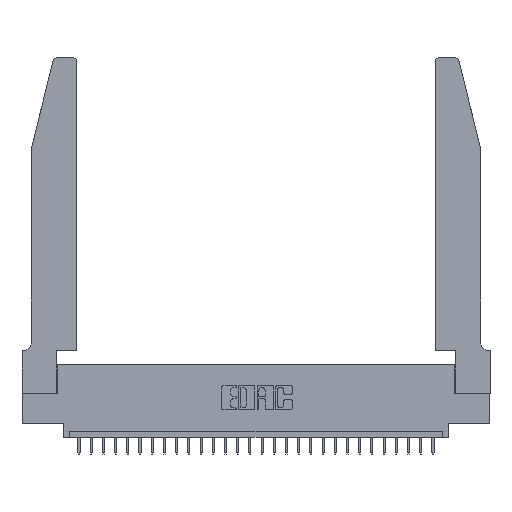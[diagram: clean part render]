
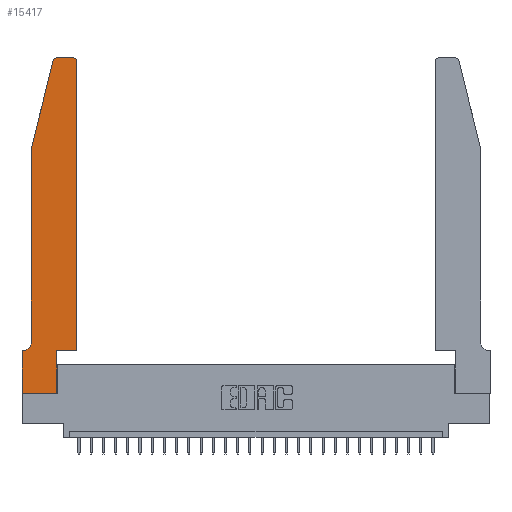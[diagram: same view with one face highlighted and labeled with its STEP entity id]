
A CAD part, top view. The second image highlights one B-rep face of the part: STEP entity #15417.
In plain terms, the highlighted planar face has unit normal (0, 0, 1).
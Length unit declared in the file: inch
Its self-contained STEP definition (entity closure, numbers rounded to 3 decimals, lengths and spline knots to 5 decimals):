
#148 = LINE ( 'NONE', #455, #2557 ) ;
#335 = VERTEX_POINT ( 'NONE', #12648 ) ;
#455 = CARTESIAN_POINT ( 'NONE',  ( 0.2865, 0.35, 0.37 ) ) ;
#881 = CARTESIAN_POINT ( 'NONE',  ( 0.4505, 0.35, 0.37 ) ) ;
#938 = CARTESIAN_POINT ( 'NONE',  ( 0., 0., 0.37 ) ) ;
#1252 = LINE ( 'NONE', #23822, #13345 ) ;
#1320 = LINE ( 'NONE', #881, #8091 ) ;
#1921 = AXIS2_PLACEMENT_3D ( 'NONE', #28984, #17761, #5962 ) ;
#2330 = EDGE_CURVE ( 'NONE', #9192, #14189, #1252, .T. ) ;
#2557 = VECTOR ( 'NONE', #20496, 39.37008 ) ;
#2582 = ORIENTED_EDGE ( 'NONE', *, *, #20068, .T. ) ;
#2652 = EDGE_CURVE ( 'NONE', #6803, #23120, #12443, .T. ) ;
#3059 = CARTESIAN_POINT ( 'NONE',  ( 0.0755, 0.42, 0.37 ) ) ;
#3950 = AXIS2_PLACEMENT_3D ( 'NONE', #7954, #5206, #16710 ) ;
#4109 = DIRECTION ( 'NONE',  ( 1., 0., 0. ) ) ;
#4267 = ORIENTED_EDGE ( 'NONE', *, *, #17699, .T. ) ;
#4570 = VECTOR ( 'NONE', #23733, 39.37008 ) ;
#5076 = EDGE_CURVE ( 'NONE', #20601, #5955, #148, .T. ) ;
#5156 = VERTEX_POINT ( 'NONE', #9600 ) ;
#5206 = DIRECTION ( 'NONE',  ( 0., 0., 1. ) ) ;
#5381 = CARTESIAN_POINT ( 'NONE',  ( 0.0055, 0.35, 0.37 ) ) ;
#5727 = CARTESIAN_POINT ( 'NONE',  ( 0.0755, 0.35, 0.37 ) ) ;
#5955 = VERTEX_POINT ( 'NONE', #24179 ) ;
#5962 = DIRECTION ( 'NONE',  ( 1., 0., 0. ) ) ;
#6500 = CARTESIAN_POINT ( 'NONE',  ( 0.2605, 2.75, 0.37 ) ) ;
#6803 = VERTEX_POINT ( 'NONE', #18201 ) ;
#6940 = DIRECTION ( 'NONE',  ( 1., 0., 0. ) ) ;
#7156 = ORIENTED_EDGE ( 'NONE', *, *, #8086, .T. ) ;
#7325 = VECTOR ( 'NONE', #28973, 39.37008 ) ;
#7926 = VERTEX_POINT ( 'NONE', #19113 ) ;
#7954 = CARTESIAN_POINT ( 'NONE',  ( 0.284, 2.72, 0.37 ) ) ;
#8086 = EDGE_CURVE ( 'NONE', #23120, #17122, #17612, .T. ) ;
#8091 = VECTOR ( 'NONE', #9861, 39.37008 ) ;
#8499 = CARTESIAN_POINT ( 'NONE',  ( 0.2865, 0., 0.37 ) ) ;
#8996 = VERTEX_POINT ( 'NONE', #24468 ) ;
#9074 = ORIENTED_EDGE ( 'NONE', *, *, #9892, .T. ) ;
#9192 = VERTEX_POINT ( 'NONE', #23008 ) ;
#9341 = EDGE_CURVE ( 'NONE', #8996, #9192, #19301, .T. ) ;
#9600 = CARTESIAN_POINT ( 'NONE',  ( 0., 0.35, 0.37 ) ) ;
#9861 = DIRECTION ( 'NONE',  ( 0., 1., 0. ) ) ;
#9892 = EDGE_CURVE ( 'NONE', #10695, #5156, #12097, .T. ) ;
#10539 = AXIS2_PLACEMENT_3D ( 'NONE', #15314, #24321, #4109 ) ;
#10695 = VERTEX_POINT ( 'NONE', #5381 ) ;
#11530 = DIRECTION ( 'NONE',  ( 0., 0., -1. ) ) ;
#12097 = LINE ( 'NONE', #5727, #20634 ) ;
#12145 = LINE ( 'NONE', #938, #12771 ) ;
#12156 = EDGE_CURVE ( 'NONE', #5955, #7926, #13893, .T. ) ;
#12443 = CIRCLE ( 'NONE', #10539, 0.03 ) ;
#12604 = ORIENTED_EDGE ( 'NONE', *, *, #18922, .T. ) ;
#12648 = CARTESIAN_POINT ( 'NONE',  ( 0., 0., 0.37 ) ) ;
#12771 = VECTOR ( 'NONE', #21150, 39.37008 ) ;
#13345 = VECTOR ( 'NONE', #21473, 39.37008 ) ;
#13556 = CARTESIAN_POINT ( 'NONE',  ( 0.4205, 2.75, 0.37 ) ) ;
#13893 = LINE ( 'NONE', #15837, #29138 ) ;
#13999 = ORIENTED_EDGE ( 'NONE', *, *, #9341, .T. ) ;
#14189 = VERTEX_POINT ( 'NONE', #3059 ) ;
#14715 = CARTESIAN_POINT ( 'NONE',  ( 0.0755, 2., 0.37 ) ) ;
#14738 = DIRECTION ( 'NONE',  ( -1., 0., 0. ) ) ;
#15314 = CARTESIAN_POINT ( 'NONE',  ( 0.4205, 2.72, 0.37 ) ) ;
#15417 = ADVANCED_FACE ( 'NONE', ( #24119 ), #26168, .T. ) ;
#15461 = ORIENTED_EDGE ( 'NONE', *, *, #5076, .T. ) ;
#15591 = VECTOR ( 'NONE', #20256, 39.37008 ) ;
#15837 = CARTESIAN_POINT ( 'NONE',  ( 0.4505, 0.35, 0.37 ) ) ;
#15863 = EDGE_LOOP ( 'NONE', ( #7156, #2582, #13999, #16639, #12604, #9074, #22399, #20000, #15461, #22987, #4267, #27259 ) ) ;
#16639 = ORIENTED_EDGE ( 'NONE', *, *, #2330, .T. ) ;
#16710 = DIRECTION ( 'NONE',  ( 1., 0., 0. ) ) ;
#17087 = AXIS2_PLACEMENT_3D ( 'NONE', #17741, #11530, #18045 ) ;
#17122 = VERTEX_POINT ( 'NONE', #22653 ) ;
#17586 = CIRCLE ( 'NONE', #3950, 0.03 ) ;
#17612 = LINE ( 'NONE', #6500, #7325 ) ;
#17699 = EDGE_CURVE ( 'NONE', #7926, #6803, #1320, .T. ) ;
#17741 = CARTESIAN_POINT ( 'NONE',  ( 0.0055, 0.42, 0.37 ) ) ;
#17761 = DIRECTION ( 'NONE',  ( 0., 0., 1. ) ) ;
#18045 = DIRECTION ( 'NONE',  ( -1., 0., 0. ) ) ;
#18201 = CARTESIAN_POINT ( 'NONE',  ( 0.4505, 2.72, 0.37 ) ) ;
#18922 = EDGE_CURVE ( 'NONE', #14189, #10695, #20853, .T. ) ;
#19113 = CARTESIAN_POINT ( 'NONE',  ( 0.4505, 0.35, 0.37 ) ) ;
#19301 = LINE ( 'NONE', #14715, #4570 ) ;
#20000 = ORIENTED_EDGE ( 'NONE', *, *, #24451, .T. ) ;
#20068 = EDGE_CURVE ( 'NONE', #17122, #8996, #17586, .T. ) ;
#20256 = DIRECTION ( 'NONE',  ( 0., -1., 0. ) ) ;
#20496 = DIRECTION ( 'NONE',  ( 0., 1., 0. ) ) ;
#20601 = VERTEX_POINT ( 'NONE', #8499 ) ;
#20634 = VECTOR ( 'NONE', #14738, 39.37008 ) ;
#20853 = CIRCLE ( 'NONE', #17087, 0.07 ) ;
#21150 = DIRECTION ( 'NONE',  ( 1., 0., 0. ) ) ;
#21473 = DIRECTION ( 'NONE',  ( 0., -1., 0. ) ) ;
#22399 = ORIENTED_EDGE ( 'NONE', *, *, #24361, .T. ) ;
#22653 = CARTESIAN_POINT ( 'NONE',  ( 0.284, 2.75, 0.37 ) ) ;
#22987 = ORIENTED_EDGE ( 'NONE', *, *, #12156, .T. ) ;
#23008 = CARTESIAN_POINT ( 'NONE',  ( 0.0755, 2., 0.37 ) ) ;
#23120 = VERTEX_POINT ( 'NONE', #13556 ) ;
#23733 = DIRECTION ( 'NONE',  ( -0.239, -0.971, 0. ) ) ;
#23822 = CARTESIAN_POINT ( 'NONE',  ( 0.0755, 2., 0.37 ) ) ;
#24119 = FACE_OUTER_BOUND ( 'NONE', #15863, .T. ) ;
#24179 = CARTESIAN_POINT ( 'NONE',  ( 0.2865, 0.35, 0.37 ) ) ;
#24321 = DIRECTION ( 'NONE',  ( 0., 0., 1. ) ) ;
#24361 = EDGE_CURVE ( 'NONE', #5156, #335, #26893, .T. ) ;
#24451 = EDGE_CURVE ( 'NONE', #335, #20601, #12145, .T. ) ;
#24468 = CARTESIAN_POINT ( 'NONE',  ( 0.25487, 2.72718, 0.37 ) ) ;
#26168 = PLANE ( 'NONE',  #1921 ) ;
#26893 = LINE ( 'NONE', #28982, #15591 ) ;
#27259 = ORIENTED_EDGE ( 'NONE', *, *, #2652, .T. ) ;
#28973 = DIRECTION ( 'NONE',  ( -1., 0., 0. ) ) ;
#28982 = CARTESIAN_POINT ( 'NONE',  ( 0., 0., 0.37 ) ) ;
#28984 = CARTESIAN_POINT ( 'NONE',  ( 0., 0.35, 0.37 ) ) ;
#29138 = VECTOR ( 'NONE', #6940, 39.37008 ) ;
